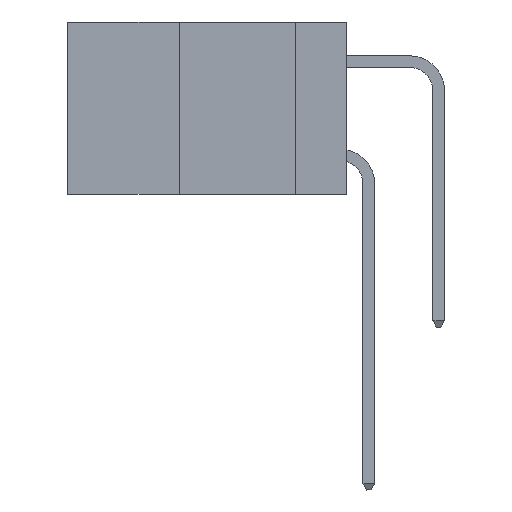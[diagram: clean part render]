
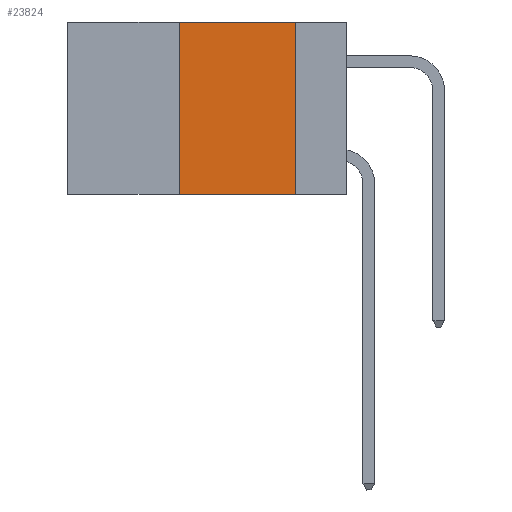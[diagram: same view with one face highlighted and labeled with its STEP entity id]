
A CAD part, left-side view. The second image highlights one B-rep face of the part: STEP entity #23824.
In plain terms, the highlighted planar face has unit normal (-1, 0, 0).
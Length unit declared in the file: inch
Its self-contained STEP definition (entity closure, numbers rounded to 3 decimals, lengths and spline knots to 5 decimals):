
#216 = PLANE ( 'NONE',  #13426 ) ;
#525 = EDGE_CURVE ( 'NONE', #3780, #17614, #8534, .T. ) ;
#3236 = EDGE_CURVE ( 'NONE', #26134, #14514, #25330, .T. ) ;
#3780 = VERTEX_POINT ( 'NONE', #22214 ) ;
#5200 = CARTESIAN_POINT ( 'NONE',  ( 0., 0.11, 0. ) ) ;
#5354 = ORIENTED_EDGE ( 'NONE', *, *, #525, .F. ) ;
#5360 = DIRECTION ( 'NONE',  ( 0., -1., 0. ) ) ;
#7142 = CARTESIAN_POINT ( 'NONE',  ( 0., 0.6, 0. ) ) ;
#8534 = LINE ( 'NONE', #20483, #18443 ) ;
#9351 = EDGE_LOOP ( 'NONE', ( #27148, #5354, #16855, #12767 ) ) ;
#11670 = EDGE_CURVE ( 'NONE', #26134, #3780, #19945, .T. ) ;
#12767 = ORIENTED_EDGE ( 'NONE', *, *, #3236, .T. ) ;
#13426 = AXIS2_PLACEMENT_3D ( 'NONE', #7142, #13634, #16125 ) ;
#13634 = DIRECTION ( 'NONE',  ( 1., 0., 0. ) ) ;
#14485 = EDGE_CURVE ( 'NONE', #17614, #14514, #24361, .T. ) ;
#14514 = VERTEX_POINT ( 'NONE', #25792 ) ;
#16125 = DIRECTION ( 'NONE',  ( 0., 0., -1. ) ) ;
#16167 = DIRECTION ( 'NONE',  ( 0., -1., 0. ) ) ;
#16855 = ORIENTED_EDGE ( 'NONE', *, *, #11670, .F. ) ;
#17138 = DIRECTION ( 'NONE',  ( 0., 0., 1. ) ) ;
#17504 = CARTESIAN_POINT ( 'NONE',  ( 0., 0.36, -0.37 ) ) ;
#17614 = VERTEX_POINT ( 'NONE', #5200 ) ;
#17972 = VECTOR ( 'NONE', #28079, 39.37008 ) ;
#18242 = CARTESIAN_POINT ( 'NONE',  ( 0., 0.6, -0.37 ) ) ;
#18443 = VECTOR ( 'NONE', #16167, 39.37008 ) ;
#19945 = LINE ( 'NONE', #25897, #25696 ) ;
#20483 = CARTESIAN_POINT ( 'NONE',  ( 0., 0.6, 0. ) ) ;
#20911 = VECTOR ( 'NONE', #5360, 39.37008 ) ;
#22214 = CARTESIAN_POINT ( 'NONE',  ( 0., 0.36, 0. ) ) ;
#23620 = CARTESIAN_POINT ( 'NONE',  ( 0., 0.11, 0. ) ) ;
#23824 = ADVANCED_FACE ( 'NONE', ( #24613 ), #216, .F. ) ;
#24361 = LINE ( 'NONE', #23620, #17972 ) ;
#24613 = FACE_OUTER_BOUND ( 'NONE', #9351, .T. ) ;
#25330 = LINE ( 'NONE', #18242, #20911 ) ;
#25696 = VECTOR ( 'NONE', #17138, 39.37008 ) ;
#25792 = CARTESIAN_POINT ( 'NONE',  ( 0., 0.11, -0.37 ) ) ;
#25897 = CARTESIAN_POINT ( 'NONE',  ( 0., 0.36, 0. ) ) ;
#26134 = VERTEX_POINT ( 'NONE', #17504 ) ;
#27148 = ORIENTED_EDGE ( 'NONE', *, *, #14485, .F. ) ;
#28079 = DIRECTION ( 'NONE',  ( 0., 0., -1. ) ) ;
